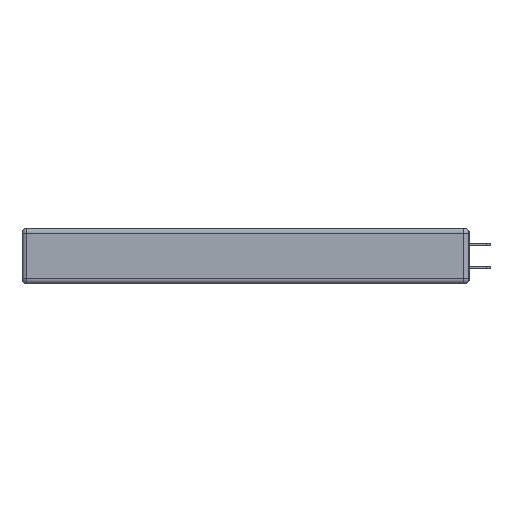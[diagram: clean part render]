
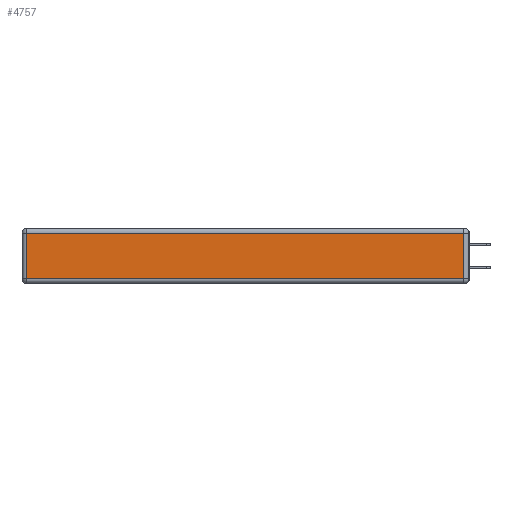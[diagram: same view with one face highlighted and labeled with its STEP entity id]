
A CAD part, left-side view. The second image highlights one B-rep face of the part: STEP entity #4757.
In plain terms, the highlighted planar face has unit normal (-1, 0, 0).
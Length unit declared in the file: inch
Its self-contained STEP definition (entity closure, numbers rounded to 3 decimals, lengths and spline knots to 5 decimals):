
#8 = CARTESIAN_POINT ( 'NONE',  ( 0., 2.72, -0.313 ) ) ;
#47 = CARTESIAN_POINT ( 'NONE',  ( 0., 0., -0.343 ) ) ;
#306 = VERTEX_POINT ( 'NONE', #16065 ) ;
#875 = DIRECTION ( 'NONE',  ( 0., -1., 0. ) ) ;
#1117 = VECTOR ( 'NONE', #15057, 39.37008 ) ;
#1364 = DIRECTION ( 'NONE',  ( 0., 0., 1. ) ) ;
#1449 = EDGE_CURVE ( 'NONE', #306, #16304, #4698, .T. ) ;
#1627 = LINE ( 'NONE', #18769, #9592 ) ;
#2460 = EDGE_CURVE ( 'NONE', #17620, #306, #1627, .T. ) ;
#2802 = ORIENTED_EDGE ( 'NONE', *, *, #8301, .T. ) ;
#2805 = EDGE_LOOP ( 'NONE', ( #16918, #15271, #2802, #9730 ) ) ;
#2919 = CARTESIAN_POINT ( 'NONE',  ( 0., 2.72, -0.343 ) ) ;
#4496 = DIRECTION ( 'NONE',  ( -1., 0., 0. ) ) ;
#4698 = LINE ( 'NONE', #14726, #11735 ) ;
#4757 = ADVANCED_FACE ( 'NONE', ( #16901 ), #10388, .T. ) ;
#5103 = LINE ( 'NONE', #2919, #1117 ) ;
#6915 = DIRECTION ( 'NONE',  ( 0., 1., 0. ) ) ;
#8301 = EDGE_CURVE ( 'NONE', #16304, #18911, #10298, .T. ) ;
#9592 = VECTOR ( 'NONE', #875, 39.37008 ) ;
#9730 = ORIENTED_EDGE ( 'NONE', *, *, #11881, .T. ) ;
#10298 = LINE ( 'NONE', #11415, #14988 ) ;
#10388 = PLANE ( 'NONE',  #14242 ) ;
#10396 = CARTESIAN_POINT ( 'NONE',  ( 0., 0.03, -0.03 ) ) ;
#10895 = CARTESIAN_POINT ( 'NONE',  ( 0., 2.72, -0.03 ) ) ;
#11415 = CARTESIAN_POINT ( 'NONE',  ( 0., 2.75, -0.03 ) ) ;
#11673 = DIRECTION ( 'NONE',  ( 0., 0., 1. ) ) ;
#11735 = VECTOR ( 'NONE', #11673, 39.37008 ) ;
#11881 = EDGE_CURVE ( 'NONE', #18911, #17620, #5103, .T. ) ;
#14242 = AXIS2_PLACEMENT_3D ( 'NONE', #47, #4496, #1364 ) ;
#14726 = CARTESIAN_POINT ( 'NONE',  ( 0., 0.03, -0.343 ) ) ;
#14988 = VECTOR ( 'NONE', #6915, 39.37008 ) ;
#15057 = DIRECTION ( 'NONE',  ( 0., 0., -1. ) ) ;
#15271 = ORIENTED_EDGE ( 'NONE', *, *, #1449, .T. ) ;
#16065 = CARTESIAN_POINT ( 'NONE',  ( 0., 0.03, -0.313 ) ) ;
#16304 = VERTEX_POINT ( 'NONE', #10396 ) ;
#16901 = FACE_OUTER_BOUND ( 'NONE', #2805, .T. ) ;
#16918 = ORIENTED_EDGE ( 'NONE', *, *, #2460, .T. ) ;
#17620 = VERTEX_POINT ( 'NONE', #8 ) ;
#18769 = CARTESIAN_POINT ( 'NONE',  ( 0., 0., -0.313 ) ) ;
#18911 = VERTEX_POINT ( 'NONE', #10895 ) ;
